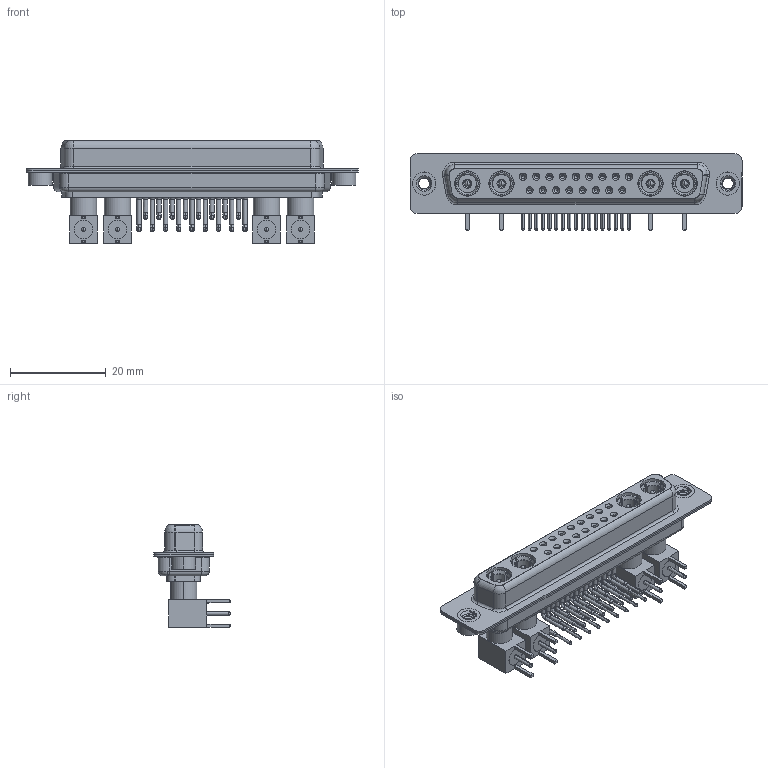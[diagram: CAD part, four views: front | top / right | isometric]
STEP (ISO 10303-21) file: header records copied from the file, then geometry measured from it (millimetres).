
FILE_DESCRIPTION (( 'STEP AP203' ), '1' );
FILE_NAME ('630-21W4640-7T2.STEP', '2022-06-08T19:20:01', ( '' ), ( '' ), 'SwSTEP 2.0', 'SolidWorks 2020', '' );
FILE_SCHEMA (( 'CONFIG_CONTROL_DESIGN' ));
Length unit declared in the file: millimetre
Products named in the file (17): 630Combo Contact Row 1; Co-Ax Plug Assy_RA; RA Back Shell; Co-Ax Plug_RA PC Tail; Pin_RA; 630Combo Shell Front_37 Contacts; 630Combo Shell Rear_37 Contacts; 630Combo Housing_21W4; 630Combo Threaded Rivet_2; Insulator Pin_Straight PC Tail; 630Combo Contact Row 2; 630-21W4640-7T2; Locking Collar; Insulator RA Pin
Assembly tree (50 placements, depth 3):
  630-21W4640-7T2
    630Combo Housing_21W4
    630Combo Shell Front_37 Contacts
    630Combo Shell Rear_37 Contacts
    630Combo Threaded Rivet_2  x2
    Co-Ax Plug Assy_RA
      Co-Ax Plug_RA PC Tail
      Insulator Pin_Straight PC Tail
      Pin_RA
      Locking Collar
      RA Back Shell
      Insulator RA Pin
    Co-Ax Plug Assy_RA
      Co-Ax Plug_RA PC Tail
      Insulator Pin_Straight PC Tail
      Pin_RA
      Locking Collar
      RA Back Shell
      Insulator RA Pin
    Co-Ax Plug Assy_RA
      Co-Ax Plug_RA PC Tail
      Insulator Pin_Straight PC Tail
      Pin_RA
      Locking Collar
      RA Back Shell
      Insulator RA Pin
    Co-Ax Plug Assy_RA
      Co-Ax Plug_RA PC Tail
      Insulator Pin_Straight PC Tail
      Pin_RA
      Locking Collar
      RA Back Shell
      Insulator RA Pin
    630Combo Contact Row 1  x9
    630Combo Contact Row 2  x8
Bounding box: 69.4 x 16 x 21.41 mm (x, y, z)
Volume: 6340.3 mm3; surface area: 15043.9 mm2
Topology: 46 solids, 46 shells, 1852 faces, 4584 edges, 2876 vertices
Faces by surface type: cylinder 788, plane 590, cone 299, torus 81, bspline 78, sphere 16
Entity records: 25928 total; most frequent: CARTESIAN_POINT 5654, DIRECTION 4034, ORIENTED_EDGE 3422, EDGE_CURVE 1711, AXIS2_PLACEMENT_3D 1667, VERTEX_POINT 1088, CIRCLE 892, EDGE_LOOP 877
